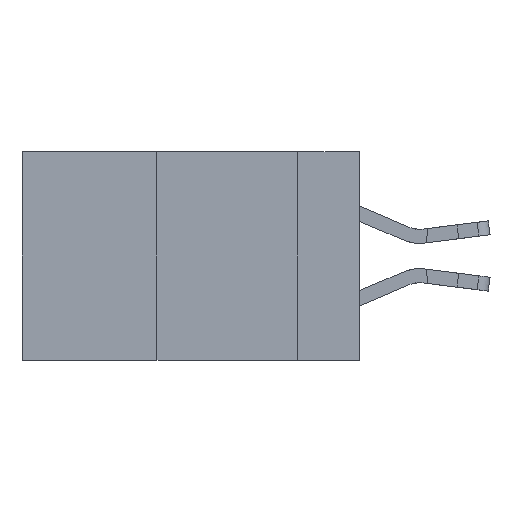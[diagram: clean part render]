
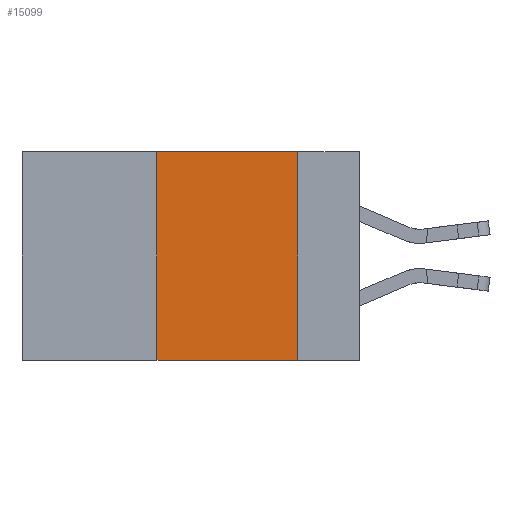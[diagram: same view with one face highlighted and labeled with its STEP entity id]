
A CAD part, left-side view. The second image highlights one B-rep face of the part: STEP entity #15099.
In plain terms, the highlighted planar face has unit normal (-1, 0, 0).
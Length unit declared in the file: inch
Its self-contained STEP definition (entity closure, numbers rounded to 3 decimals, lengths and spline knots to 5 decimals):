
#1129 = CARTESIAN_POINT ( 'NONE',  ( 0., 0.36, 0. ) ) ;
#1470 = VERTEX_POINT ( 'NONE', #22232 ) ;
#1591 = VERTEX_POINT ( 'NONE', #12117 ) ;
#1870 = DIRECTION ( 'NONE',  ( 0., 0., -1. ) ) ;
#3659 = VERTEX_POINT ( 'NONE', #4887 ) ;
#3934 = CARTESIAN_POINT ( 'NONE',  ( 0., 0.11, 0. ) ) ;
#4125 = AXIS2_PLACEMENT_3D ( 'NONE', #25193, #5478, #19384 ) ;
#4310 = CARTESIAN_POINT ( 'NONE',  ( 0., 0.6, -0.37 ) ) ;
#4398 = EDGE_CURVE ( 'NONE', #3659, #7712, #15870, .T. ) ;
#4887 = CARTESIAN_POINT ( 'NONE',  ( 0., 0.36, -0.37 ) ) ;
#4921 = DIRECTION ( 'NONE',  ( 0., -1., 0. ) ) ;
#5478 = DIRECTION ( 'NONE',  ( 1., 0., 0. ) ) ;
#5610 = VECTOR ( 'NONE', #1870, 39.37008 ) ;
#7712 = VERTEX_POINT ( 'NONE', #10166 ) ;
#8984 = ORIENTED_EDGE ( 'NONE', *, *, #13564, .F. ) ;
#10166 = CARTESIAN_POINT ( 'NONE',  ( 0., 0.11, -0.37 ) ) ;
#10743 = CARTESIAN_POINT ( 'NONE',  ( 0., 0.6, 0. ) ) ;
#11688 = EDGE_CURVE ( 'NONE', #3659, #1591, #14650, .T. ) ;
#12117 = CARTESIAN_POINT ( 'NONE',  ( 0., 0.36, 0. ) ) ;
#12657 = EDGE_CURVE ( 'NONE', #1470, #7712, #16129, .T. ) ;
#13532 = ORIENTED_EDGE ( 'NONE', *, *, #4398, .T. ) ;
#13564 = EDGE_CURVE ( 'NONE', #1591, #1470, #16081, .T. ) ;
#14650 = LINE ( 'NONE', #1129, #23331 ) ;
#15099 = ADVANCED_FACE ( 'NONE', ( #21373 ), #17386, .F. ) ;
#15481 = VECTOR ( 'NONE', #16735, 39.37008 ) ;
#15870 = LINE ( 'NONE', #4310, #16500 ) ;
#16081 = LINE ( 'NONE', #10743, #15481 ) ;
#16129 = LINE ( 'NONE', #3934, #5610 ) ;
#16500 = VECTOR ( 'NONE', #4921, 39.37008 ) ;
#16735 = DIRECTION ( 'NONE',  ( 0., -1., 0. ) ) ;
#17386 = PLANE ( 'NONE',  #4125 ) ;
#19384 = DIRECTION ( 'NONE',  ( 0., 0., -1. ) ) ;
#19494 = ORIENTED_EDGE ( 'NONE', *, *, #11688, .F. ) ;
#19696 = EDGE_LOOP ( 'NONE', ( #19883, #8984, #19494, #13532 ) ) ;
#19883 = ORIENTED_EDGE ( 'NONE', *, *, #12657, .F. ) ;
#21373 = FACE_OUTER_BOUND ( 'NONE', #19696, .T. ) ;
#22232 = CARTESIAN_POINT ( 'NONE',  ( 0., 0.11, 0. ) ) ;
#23331 = VECTOR ( 'NONE', #24896, 39.37008 ) ;
#24896 = DIRECTION ( 'NONE',  ( 0., 0., 1. ) ) ;
#25193 = CARTESIAN_POINT ( 'NONE',  ( 0., 0.6, 0. ) ) ;
